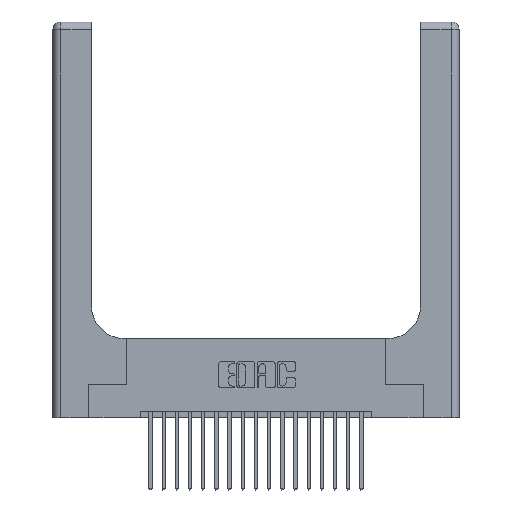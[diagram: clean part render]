
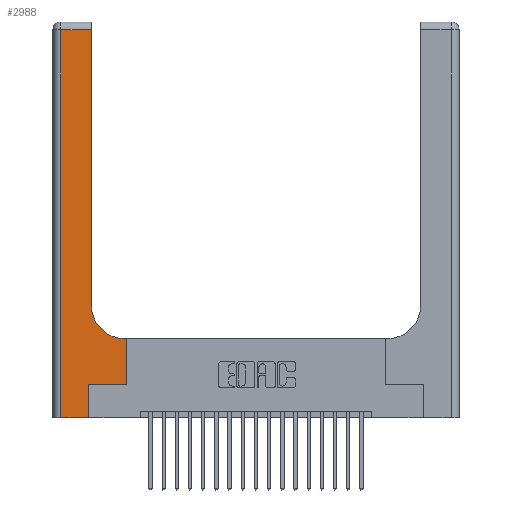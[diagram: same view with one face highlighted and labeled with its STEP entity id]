
A CAD part, top view. The second image highlights one B-rep face of the part: STEP entity #2988.
In plain terms, the highlighted planar face has unit normal (0, 0, 1).
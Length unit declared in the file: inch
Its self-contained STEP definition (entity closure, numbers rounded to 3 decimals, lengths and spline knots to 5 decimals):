
#492 = DIRECTION ( 'NONE',  ( -1., 0., 0. ) ) ;
#608 = ORIENTED_EDGE ( 'NONE', *, *, #13867, .T. ) ;
#644 = EDGE_CURVE ( 'NONE', #7308, #14778, #7751, .T. ) ;
#780 = EDGE_CURVE ( 'NONE', #1416, #12608, #19595, .T. ) ;
#920 = DIRECTION ( 'NONE',  ( 0., 1., 0. ) ) ;
#1180 = CARTESIAN_POINT ( 'NONE',  ( 0.5585, 0.25, 0.37 ) ) ;
#1416 = VERTEX_POINT ( 'NONE', #2819 ) ;
#1511 = PLANE ( 'NONE',  #12034 ) ;
#2197 = ORIENTED_EDGE ( 'NONE', *, *, #9848, .T. ) ;
#2819 = CARTESIAN_POINT ( 'NONE',  ( 0.5585, 0.25, 0.37 ) ) ;
#2988 = ADVANCED_FACE ( 'NONE', ( #4896 ), #1511, .F. ) ;
#3152 = VECTOR ( 'NONE', #8706, 39.37008 ) ;
#3253 = DIRECTION ( 'NONE',  ( -1., 0., 0. ) ) ;
#3315 = CARTESIAN_POINT ( 'NONE',  ( 0.269, 0., 0.37 ) ) ;
#3449 = DIRECTION ( 'NONE',  ( 0., 0., -1. ) ) ;
#4374 = EDGE_CURVE ( 'NONE', #14778, #11405, #8047, .T. ) ;
#4503 = LINE ( 'NONE', #19858, #17464 ) ;
#4673 = CARTESIAN_POINT ( 'NONE',  ( 0.5585, 0.6, 0.37 ) ) ;
#4870 = VERTEX_POINT ( 'NONE', #16870 ) ;
#4896 = FACE_OUTER_BOUND ( 'NONE', #18898, .T. ) ;
#5128 = CARTESIAN_POINT ( 'NONE',  ( 0., 0., 0.37 ) ) ;
#5404 = ORIENTED_EDGE ( 'NONE', *, *, #6143, .T. ) ;
#5783 = CARTESIAN_POINT ( 'NONE',  ( 0.2915, 3., 0.37 ) ) ;
#5946 = ORIENTED_EDGE ( 'NONE', *, *, #18259, .T. ) ;
#6143 = EDGE_CURVE ( 'NONE', #15703, #1416, #4503, .T. ) ;
#6241 = ORIENTED_EDGE ( 'NONE', *, *, #7447, .T. ) ;
#6676 = CARTESIAN_POINT ( 'NONE',  ( 0., 3., 0.37 ) ) ;
#6866 = VECTOR ( 'NONE', #7079, 39.37008 ) ;
#7079 = DIRECTION ( 'NONE',  ( -1., 0., 0. ) ) ;
#7308 = VERTEX_POINT ( 'NONE', #10169 ) ;
#7447 = EDGE_CURVE ( 'NONE', #4870, #7308, #20266, .T. ) ;
#7751 = LINE ( 'NONE', #7863, #3152 ) ;
#7797 = LINE ( 'NONE', #10830, #12860 ) ;
#7858 = ORIENTED_EDGE ( 'NONE', *, *, #780, .T. ) ;
#7863 = CARTESIAN_POINT ( 'NONE',  ( 0.06, 3., 0.37 ) ) ;
#8047 = LINE ( 'NONE', #5128, #15960 ) ;
#8184 = CIRCLE ( 'NONE', #19799, 0.25 ) ;
#8706 = DIRECTION ( 'NONE',  ( 0., -1., 0. ) ) ;
#8750 = DIRECTION ( 'NONE',  ( 0., 1., 0. ) ) ;
#9848 = EDGE_CURVE ( 'NONE', #12608, #20670, #7797, .T. ) ;
#10169 = CARTESIAN_POINT ( 'NONE',  ( 0.06, 2.94, 0.37 ) ) ;
#10174 = VECTOR ( 'NONE', #920, 39.37008 ) ;
#10207 = CARTESIAN_POINT ( 'NONE',  ( 0.2915, 0.85, 0.37 ) ) ;
#10713 = CARTESIAN_POINT ( 'NONE',  ( 0.06, 0., 0.37 ) ) ;
#10830 = CARTESIAN_POINT ( 'NONE',  ( 0.2915, 0.6, 0.37 ) ) ;
#11405 = VERTEX_POINT ( 'NONE', #3315 ) ;
#12034 = AXIS2_PLACEMENT_3D ( 'NONE', #6676, #13498, #3253 ) ;
#12504 = LINE ( 'NONE', #20460, #16950 ) ;
#12608 = VERTEX_POINT ( 'NONE', #4673 ) ;
#12725 = EDGE_CURVE ( 'NONE', #11405, #15703, #12504, .T. ) ;
#12860 = VECTOR ( 'NONE', #492, 39.37008 ) ;
#12959 = CARTESIAN_POINT ( 'NONE',  ( 0.269, 0.25, 0.37 ) ) ;
#13347 = ORIENTED_EDGE ( 'NONE', *, *, #12725, .T. ) ;
#13498 = DIRECTION ( 'NONE',  ( 0., 0., -1. ) ) ;
#13674 = CARTESIAN_POINT ( 'NONE',  ( 0.5415, 0.85, 0.37 ) ) ;
#13867 = EDGE_CURVE ( 'NONE', #20670, #14565, #8184, .T. ) ;
#14565 = VERTEX_POINT ( 'NONE', #10207 ) ;
#14778 = VERTEX_POINT ( 'NONE', #10713 ) ;
#15343 = DIRECTION ( 'NONE',  ( 1., 0., 0. ) ) ;
#15447 = VECTOR ( 'NONE', #17611, 39.37008 ) ;
#15514 = CARTESIAN_POINT ( 'NONE',  ( 0., 2.94, 0.37 ) ) ;
#15703 = VERTEX_POINT ( 'NONE', #12959 ) ;
#15960 = VECTOR ( 'NONE', #20274, 39.37008 ) ;
#16465 = ORIENTED_EDGE ( 'NONE', *, *, #644, .T. ) ;
#16706 = ORIENTED_EDGE ( 'NONE', *, *, #4374, .T. ) ;
#16870 = CARTESIAN_POINT ( 'NONE',  ( 0.2915, 2.94, 0.37 ) ) ;
#16950 = VECTOR ( 'NONE', #8750, 39.37008 ) ;
#17464 = VECTOR ( 'NONE', #21473, 39.37008 ) ;
#17611 = DIRECTION ( 'NONE',  ( 0., 1., 0. ) ) ;
#18259 = EDGE_CURVE ( 'NONE', #14565, #4870, #19870, .T. ) ;
#18898 = EDGE_LOOP ( 'NONE', ( #5946, #6241, #16465, #16706, #13347, #5404, #7858, #2197, #608 ) ) ;
#19595 = LINE ( 'NONE', #1180, #10174 ) ;
#19773 = CARTESIAN_POINT ( 'NONE',  ( 0.5415, 0.6, 0.37 ) ) ;
#19799 = AXIS2_PLACEMENT_3D ( 'NONE', #13674, #3449, #15343 ) ;
#19858 = CARTESIAN_POINT ( 'NONE',  ( 0.269, 0.25, 0.37 ) ) ;
#19870 = LINE ( 'NONE', #5783, #15447 ) ;
#20266 = LINE ( 'NONE', #15514, #6866 ) ;
#20274 = DIRECTION ( 'NONE',  ( 1., 0., 0. ) ) ;
#20460 = CARTESIAN_POINT ( 'NONE',  ( 0.269, 0., 0.37 ) ) ;
#20670 = VERTEX_POINT ( 'NONE', #19773 ) ;
#21473 = DIRECTION ( 'NONE',  ( 1., 0., 0. ) ) ;
